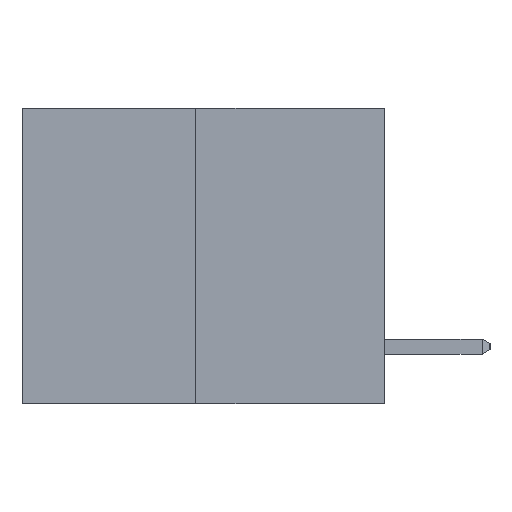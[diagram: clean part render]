
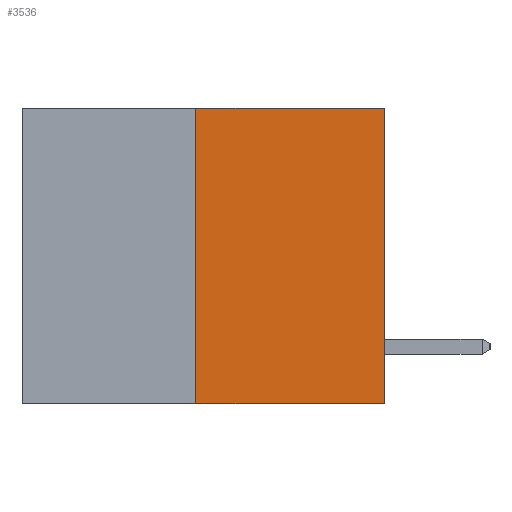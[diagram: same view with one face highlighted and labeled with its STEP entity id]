
A CAD part, left-side view. The second image highlights one B-rep face of the part: STEP entity #3536.
In plain terms, the highlighted planar face has unit normal (-1, 0, 0).
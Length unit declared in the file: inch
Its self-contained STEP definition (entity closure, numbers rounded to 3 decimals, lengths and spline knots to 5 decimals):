
#811 = DIRECTION ( 'NONE',  ( 1., 0., 0. ) ) ;
#829 = EDGE_CURVE ( 'NONE', #25144, #5244, #1105, .T. ) ;
#1105 = LINE ( 'NONE', #8643, #14393 ) ;
#1232 = CARTESIAN_POINT ( 'NONE',  ( 0., 0.6, 0. ) ) ;
#1379 = VERTEX_POINT ( 'NONE', #21134 ) ;
#1435 = LINE ( 'NONE', #1232, #18991 ) ;
#3490 = ORIENTED_EDGE ( 'NONE', *, *, #3743, .T. ) ;
#3528 = CARTESIAN_POINT ( 'NONE',  ( 0., 0.312, 0. ) ) ;
#3536 = ADVANCED_FACE ( 'NONE', ( #21864 ), #10606, .F. ) ;
#3743 = EDGE_CURVE ( 'NONE', #25144, #1379, #11217, .T. ) ;
#5196 = AXIS2_PLACEMENT_3D ( 'NONE', #24319, #811, #18598 ) ;
#5244 = VERTEX_POINT ( 'NONE', #3528 ) ;
#6882 = LINE ( 'NONE', #20971, #24676 ) ;
#7011 = DIRECTION ( 'NONE',  ( 0., -1., 0. ) ) ;
#7678 = DIRECTION ( 'NONE',  ( 0., -1., 0. ) ) ;
#8643 = CARTESIAN_POINT ( 'NONE',  ( 0., 0.312, -0.49 ) ) ;
#9384 = VERTEX_POINT ( 'NONE', #18509 ) ;
#10493 = CARTESIAN_POINT ( 'NONE',  ( 0., 0.312, -0.49 ) ) ;
#10606 = PLANE ( 'NONE',  #5196 ) ;
#11217 = LINE ( 'NONE', #11638, #11845 ) ;
#11638 = CARTESIAN_POINT ( 'NONE',  ( 0., 0.6, -0.49 ) ) ;
#11845 = VECTOR ( 'NONE', #7678, 39.37008 ) ;
#12082 = EDGE_CURVE ( 'NONE', #1379, #9384, #6882, .T. ) ;
#14393 = VECTOR ( 'NONE', #18359, 39.37008 ) ;
#15988 = EDGE_LOOP ( 'NONE', ( #18903, #3490, #20813, #21170 ) ) ;
#18359 = DIRECTION ( 'NONE',  ( 0., 0., 1. ) ) ;
#18509 = CARTESIAN_POINT ( 'NONE',  ( 0., 0., 0. ) ) ;
#18598 = DIRECTION ( 'NONE',  ( 0., 0., -1. ) ) ;
#18903 = ORIENTED_EDGE ( 'NONE', *, *, #829, .F. ) ;
#18991 = VECTOR ( 'NONE', #7011, 39.37008 ) ;
#20813 = ORIENTED_EDGE ( 'NONE', *, *, #12082, .T. ) ;
#20971 = CARTESIAN_POINT ( 'NONE',  ( 0., 0., 0. ) ) ;
#21134 = CARTESIAN_POINT ( 'NONE',  ( 0., 0., -0.49 ) ) ;
#21138 = DIRECTION ( 'NONE',  ( 0., 0., 1. ) ) ;
#21170 = ORIENTED_EDGE ( 'NONE', *, *, #24128, .F. ) ;
#21864 = FACE_OUTER_BOUND ( 'NONE', #15988, .T. ) ;
#24128 = EDGE_CURVE ( 'NONE', #5244, #9384, #1435, .T. ) ;
#24319 = CARTESIAN_POINT ( 'NONE',  ( 0., 0.6, 0. ) ) ;
#24676 = VECTOR ( 'NONE', #21138, 39.37008 ) ;
#25144 = VERTEX_POINT ( 'NONE', #10493 ) ;
